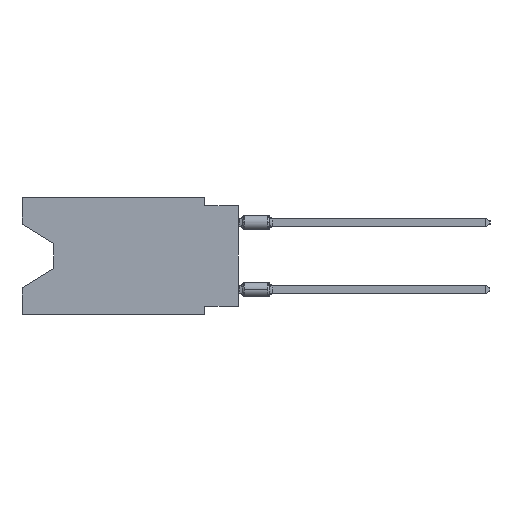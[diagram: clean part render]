
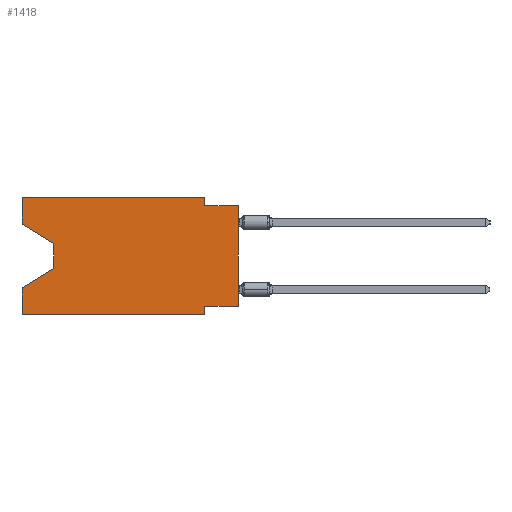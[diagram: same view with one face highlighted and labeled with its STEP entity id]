
A CAD part, left-side view. The second image highlights one B-rep face of the part: STEP entity #1418.
In plain terms, the highlighted planar face has unit normal (-1, 0, 0).
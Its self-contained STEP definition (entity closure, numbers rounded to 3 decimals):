
#127 = EDGE_CURVE ( 'NONE', #19657, #18455, #11381, .T. ) ;
#527 = VECTOR ( 'NONE', #5828, 1000. ) ;
#888 = CARTESIAN_POINT ( 'NONE',  ( 0., 16.383, -8.89 ) ) ;
#1094 = DIRECTION ( 'NONE',  ( 0., 0., -1. ) ) ;
#1418 = ADVANCED_FACE ( 'NONE', ( #20972 ), #19009, .F. ) ;
#1785 = EDGE_CURVE ( 'NONE', #10140, #23011, #11493, .T. ) ;
#1854 = ORIENTED_EDGE ( 'NONE', *, *, #19776, .T. ) ;
#1932 = DIRECTION ( 'NONE',  ( 0., 0., 1. ) ) ;
#1969 = CARTESIAN_POINT ( 'NONE',  ( 0., 2.54, 0. ) ) ;
#1973 = VERTEX_POINT ( 'NONE', #13450 ) ;
#2007 = VERTEX_POINT ( 'NONE', #15732 ) ;
#2061 = ORIENTED_EDGE ( 'NONE', *, *, #10880, .F. ) ;
#2069 = LINE ( 'NONE', #5972, #18830 ) ;
#2266 = DIRECTION ( 'NONE',  ( 0., 0., -1. ) ) ;
#2767 = CARTESIAN_POINT ( 'NONE',  ( 0., 2.54, -8.255 ) ) ;
#2878 = DIRECTION ( 'NONE',  ( 0., -1., 0. ) ) ;
#3065 = ORIENTED_EDGE ( 'NONE', *, *, #127, .F. ) ;
#3080 = VECTOR ( 'NONE', #18962, 1000. ) ;
#3202 = VECTOR ( 'NONE', #18751, 1000. ) ;
#3421 = EDGE_CURVE ( 'NONE', #6397, #24985, #21033, .T. ) ;
#3543 = CARTESIAN_POINT ( 'NONE',  ( 0., 13.97, -3.505 ) ) ;
#4196 = CARTESIAN_POINT ( 'NONE',  ( 0., 2.54, -0.635 ) ) ;
#4349 = DIRECTION ( 'NONE',  ( 0., 0., 1. ) ) ;
#4678 = CARTESIAN_POINT ( 'NONE',  ( 0., 0., -0.635 ) ) ;
#4873 = CARTESIAN_POINT ( 'NONE',  ( 0., 16.383, 0. ) ) ;
#5297 = EDGE_LOOP ( 'NONE', ( #1854, #22993, #10577, #25049, #18059, #9094, #3065, #24119, #14584, #2061, #7781, #17678 ) ) ;
#5609 = DIRECTION ( 'NONE',  ( 0., -0.855, -0.519 ) ) ;
#5828 = DIRECTION ( 'NONE',  ( 0., 0., -1. ) ) ;
#5972 = CARTESIAN_POINT ( 'NONE',  ( 0., 16.383, 0. ) ) ;
#6397 = VERTEX_POINT ( 'NONE', #4873 ) ;
#6854 = EDGE_CURVE ( 'NONE', #19657, #1973, #17001, .T. ) ;
#7433 = CARTESIAN_POINT ( 'NONE',  ( 0., 13.97, -5.385 ) ) ;
#7446 = LINE ( 'NONE', #15558, #15126 ) ;
#7449 = CARTESIAN_POINT ( 'NONE',  ( 0., 0., -8.255 ) ) ;
#7453 = DIRECTION ( 'NONE',  ( 0., 0., -1. ) ) ;
#7578 = LINE ( 'NONE', #3543, #23049 ) ;
#7689 = DIRECTION ( 'NONE',  ( 0., 0.855, -0.519 ) ) ;
#7781 = ORIENTED_EDGE ( 'NONE', *, *, #3421, .F. ) ;
#7787 = CARTESIAN_POINT ( 'NONE',  ( 0., 16.383, -2.038 ) ) ;
#8681 = CARTESIAN_POINT ( 'NONE',  ( 0., 16.383, -6.852 ) ) ;
#8723 = DIRECTION ( 'NONE',  ( 0., -1., 0. ) ) ;
#9094 = ORIENTED_EDGE ( 'NONE', *, *, #19025, .F. ) ;
#9455 = VECTOR ( 'NONE', #8723, 1000. ) ;
#9530 = EDGE_CURVE ( 'NONE', #10130, #1973, #22854, .T. ) ;
#9532 = VECTOR ( 'NONE', #25115, 1000. ) ;
#9756 = EDGE_CURVE ( 'NONE', #2007, #23011, #14548, .T. ) ;
#10130 = VERTEX_POINT ( 'NONE', #4196 ) ;
#10140 = VERTEX_POINT ( 'NONE', #20403 ) ;
#10577 = ORIENTED_EDGE ( 'NONE', *, *, #1785, .T. ) ;
#10742 = AXIS2_PLACEMENT_3D ( 'NONE', #25068, #22690, #1094 ) ;
#10749 = CARTESIAN_POINT ( 'NONE',  ( 0., 16.383, 0. ) ) ;
#10880 = EDGE_CURVE ( 'NONE', #24985, #10130, #21616, .T. ) ;
#11146 = VECTOR ( 'NONE', #4349, 1000. ) ;
#11381 = LINE ( 'NONE', #7449, #3202 ) ;
#11461 = LINE ( 'NONE', #888, #9532 ) ;
#11493 = LINE ( 'NONE', #7433, #12002 ) ;
#12002 = VECTOR ( 'NONE', #7689, 1000. ) ;
#12088 = VERTEX_POINT ( 'NONE', #7787 ) ;
#12731 = CARTESIAN_POINT ( 'NONE',  ( 0., 0., -8.255 ) ) ;
#13074 = CARTESIAN_POINT ( 'NONE',  ( 0., 0., 0. ) ) ;
#13175 = EDGE_CURVE ( 'NONE', #2007, #19272, #11461, .T. ) ;
#13450 = CARTESIAN_POINT ( 'NONE',  ( 0., 0., -0.635 ) ) ;
#14548 = LINE ( 'NONE', #10749, #11146 ) ;
#14584 = ORIENTED_EDGE ( 'NONE', *, *, #9530, .F. ) ;
#15126 = VECTOR ( 'NONE', #5609, 1000. ) ;
#15265 = LINE ( 'NONE', #17609, #527 ) ;
#15558 = CARTESIAN_POINT ( 'NONE',  ( 0., 16.383, -2.038 ) ) ;
#15732 = CARTESIAN_POINT ( 'NONE',  ( 0., 16.383, -8.89 ) ) ;
#17001 = LINE ( 'NONE', #13074, #3080 ) ;
#17609 = CARTESIAN_POINT ( 'NONE',  ( 0., 2.54, -8.89 ) ) ;
#17678 = ORIENTED_EDGE ( 'NONE', *, *, #23579, .F. ) ;
#18059 = ORIENTED_EDGE ( 'NONE', *, *, #13175, .T. ) ;
#18332 = VECTOR ( 'NONE', #2878, 1000. ) ;
#18455 = VERTEX_POINT ( 'NONE', #2767 ) ;
#18686 = CARTESIAN_POINT ( 'NONE',  ( 0., 16.383, 0. ) ) ;
#18751 = DIRECTION ( 'NONE',  ( 0., 1., 0. ) ) ;
#18830 = VECTOR ( 'NONE', #1932, 1000. ) ;
#18962 = DIRECTION ( 'NONE',  ( 0., 0., 1. ) ) ;
#19009 = PLANE ( 'NONE',  #10742 ) ;
#19025 = EDGE_CURVE ( 'NONE', #18455, #19272, #15265, .T. ) ;
#19272 = VERTEX_POINT ( 'NONE', #22833 ) ;
#19657 = VERTEX_POINT ( 'NONE', #12731 ) ;
#19776 = EDGE_CURVE ( 'NONE', #12088, #24229, #7446, .T. ) ;
#20166 = CARTESIAN_POINT ( 'NONE',  ( 0., 2.54, 0. ) ) ;
#20403 = CARTESIAN_POINT ( 'NONE',  ( 0., 13.97, -5.385 ) ) ;
#20972 = FACE_OUTER_BOUND ( 'NONE', #5297, .T. ) ;
#21033 = LINE ( 'NONE', #18686, #18332 ) ;
#21616 = LINE ( 'NONE', #20166, #23920 ) ;
#22690 = DIRECTION ( 'NONE',  ( 1., 0., 0. ) ) ;
#22817 = CARTESIAN_POINT ( 'NONE',  ( 0., 13.97, -3.505 ) ) ;
#22833 = CARTESIAN_POINT ( 'NONE',  ( 0., 2.54, -8.89 ) ) ;
#22854 = LINE ( 'NONE', #4678, #9455 ) ;
#22993 = ORIENTED_EDGE ( 'NONE', *, *, #24857, .T. ) ;
#23011 = VERTEX_POINT ( 'NONE', #8681 ) ;
#23049 = VECTOR ( 'NONE', #7453, 1000. ) ;
#23579 = EDGE_CURVE ( 'NONE', #12088, #6397, #2069, .T. ) ;
#23920 = VECTOR ( 'NONE', #2266, 1000. ) ;
#24119 = ORIENTED_EDGE ( 'NONE', *, *, #6854, .T. ) ;
#24229 = VERTEX_POINT ( 'NONE', #22817 ) ;
#24857 = EDGE_CURVE ( 'NONE', #24229, #10140, #7578, .T. ) ;
#24985 = VERTEX_POINT ( 'NONE', #1969 ) ;
#25049 = ORIENTED_EDGE ( 'NONE', *, *, #9756, .F. ) ;
#25068 = CARTESIAN_POINT ( 'NONE',  ( 0., 16.383, 0. ) ) ;
#25115 = DIRECTION ( 'NONE',  ( 0., -1., 0. ) ) ;
